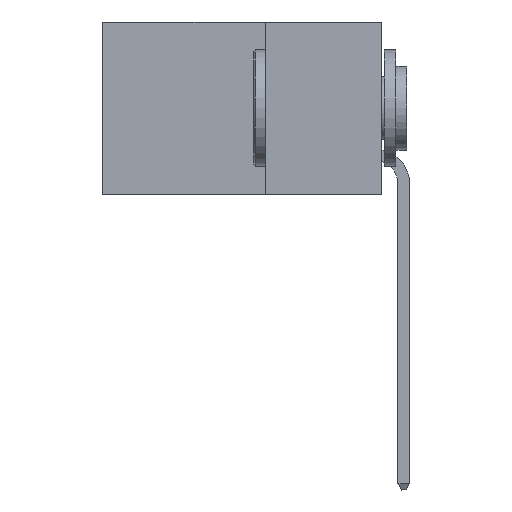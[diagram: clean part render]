
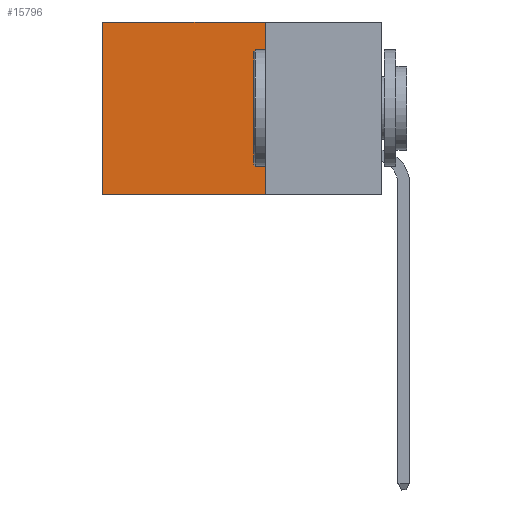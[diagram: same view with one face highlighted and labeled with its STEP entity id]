
A CAD part, left-side view. The second image highlights one B-rep face of the part: STEP entity #15796.
In plain terms, the highlighted planar face has unit normal (-1, 0, 0).
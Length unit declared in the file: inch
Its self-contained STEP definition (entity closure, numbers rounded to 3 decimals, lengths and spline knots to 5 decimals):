
#758 = VECTOR ( 'NONE', #2931, 39.37008 ) ;
#1463 = DIRECTION ( 'NONE',  ( 0., 0., -1. ) ) ;
#2931 = DIRECTION ( 'NONE',  ( 0., 0., -1. ) ) ;
#3136 = VECTOR ( 'NONE', #1463, 39.37008 ) ;
#3571 = FACE_OUTER_BOUND ( 'NONE', #18187, .T. ) ;
#3823 = CARTESIAN_POINT ( 'NONE',  ( 0.2875, 0.25, 0. ) ) ;
#3978 = DIRECTION ( 'NONE',  ( 0., 1., 0. ) ) ;
#4232 = CARTESIAN_POINT ( 'NONE',  ( 0.2875, 0.6, 0. ) ) ;
#4772 = VERTEX_POINT ( 'NONE', #8372 ) ;
#5230 = VECTOR ( 'NONE', #3978, 39.37008 ) ;
#5466 = EDGE_CURVE ( 'NONE', #15623, #16843, #6839, .T. ) ;
#5680 = ORIENTED_EDGE ( 'NONE', *, *, #12782, .T. ) ;
#5794 = CARTESIAN_POINT ( 'NONE',  ( 0.2875, 0.25, 0. ) ) ;
#6231 = CARTESIAN_POINT ( 'NONE',  ( 0.2875, 0.25, 0. ) ) ;
#6790 = EDGE_CURVE ( 'NONE', #4772, #16843, #9911, .T. ) ;
#6839 = LINE ( 'NONE', #8215, #5230 ) ;
#7173 = CARTESIAN_POINT ( 'NONE',  ( 0.2875, 0.25, -0.37 ) ) ;
#7260 = ORIENTED_EDGE ( 'NONE', *, *, #6790, .T. ) ;
#7759 = VECTOR ( 'NONE', #18487, 39.37008 ) ;
#8215 = CARTESIAN_POINT ( 'NONE',  ( 0.2875, 0.25, -0.37 ) ) ;
#8286 = VERTEX_POINT ( 'NONE', #5794 ) ;
#8372 = CARTESIAN_POINT ( 'NONE',  ( 0.2875, 0.6, 0. ) ) ;
#8508 = LINE ( 'NONE', #3823, #758 ) ;
#8949 = DIRECTION ( 'NONE',  ( 0., 0., -1. ) ) ;
#9400 = AXIS2_PLACEMENT_3D ( 'NONE', #6231, #17712, #8949 ) ;
#9911 = LINE ( 'NONE', #4232, #3136 ) ;
#10172 = EDGE_CURVE ( 'NONE', #8286, #15623, #8508, .T. ) ;
#10412 = PLANE ( 'NONE',  #9400 ) ;
#11393 = ORIENTED_EDGE ( 'NONE', *, *, #5466, .F. ) ;
#12782 = EDGE_CURVE ( 'NONE', #8286, #4772, #14277, .T. ) ;
#14277 = LINE ( 'NONE', #18677, #7759 ) ;
#15623 = VERTEX_POINT ( 'NONE', #7173 ) ;
#15796 = ADVANCED_FACE ( 'NONE', ( #3571 ), #10412, .F. ) ;
#15978 = ORIENTED_EDGE ( 'NONE', *, *, #10172, .F. ) ;
#16843 = VERTEX_POINT ( 'NONE', #17475 ) ;
#17475 = CARTESIAN_POINT ( 'NONE',  ( 0.2875, 0.6, -0.37 ) ) ;
#17712 = DIRECTION ( 'NONE',  ( 1., 0., 0. ) ) ;
#18187 = EDGE_LOOP ( 'NONE', ( #7260, #11393, #15978, #5680 ) ) ;
#18487 = DIRECTION ( 'NONE',  ( 0., 1., 0. ) ) ;
#18677 = CARTESIAN_POINT ( 'NONE',  ( 0.2875, 0.25, 0. ) ) ;
